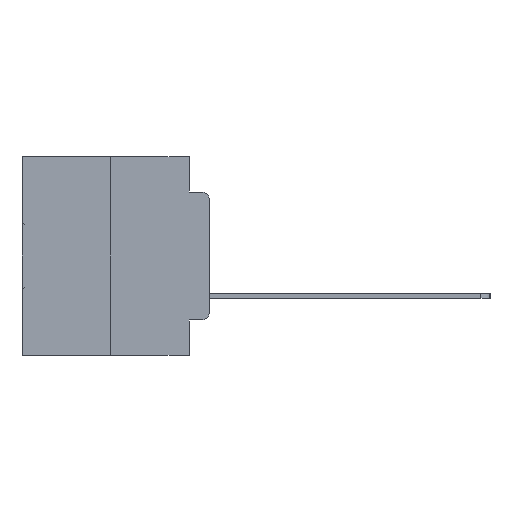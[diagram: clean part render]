
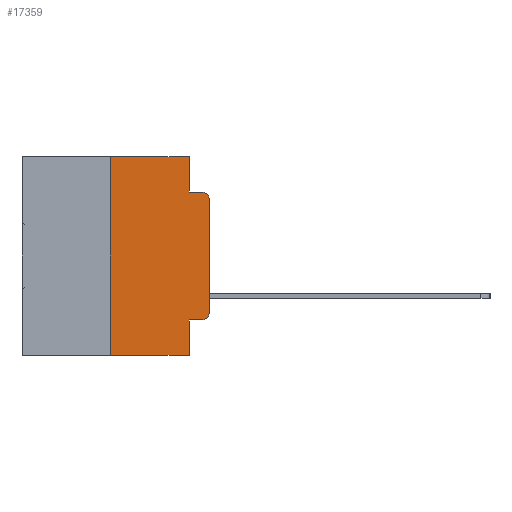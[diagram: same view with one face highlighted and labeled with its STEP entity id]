
A CAD part, left-side view. The second image highlights one B-rep face of the part: STEP entity #17359.
In plain terms, the highlighted planar face has unit normal (-1, 0, 0).
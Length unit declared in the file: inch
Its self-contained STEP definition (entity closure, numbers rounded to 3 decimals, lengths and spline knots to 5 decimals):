
#674 = EDGE_CURVE ( 'NONE', #1802, #11929, #8612, .T. ) ;
#1368 = CARTESIAN_POINT ( 'NONE',  ( 0., 0.473, 0. ) ) ;
#1500 = CARTESIAN_POINT ( 'NONE',  ( 0., 0.25, 0. ) ) ;
#1729 = CARTESIAN_POINT ( 'NONE',  ( 0., 0.02, -0.1085 ) ) ;
#1802 = VERTEX_POINT ( 'NONE', #5630 ) ;
#1898 = VERTEX_POINT ( 'NONE', #11949 ) ;
#2174 = VERTEX_POINT ( 'NONE', #17420 ) ;
#2184 = ORIENTED_EDGE ( 'NONE', *, *, #27439, .F. ) ;
#2606 = VECTOR ( 'NONE', #14664, 39.37008 ) ;
#2814 = CARTESIAN_POINT ( 'NONE',  ( 0., 0.051, 0. ) ) ;
#2825 = ORIENTED_EDGE ( 'NONE', *, *, #14005, .F. ) ;
#3076 = CARTESIAN_POINT ( 'NONE',  ( 0., 0.051, -0.0885 ) ) ;
#3479 = VERTEX_POINT ( 'NONE', #28810 ) ;
#3806 = DIRECTION ( 'NONE',  ( 0., 0., -1. ) ) ;
#3943 = CIRCLE ( 'NONE', #24293, 0.02 ) ;
#4190 = DIRECTION ( 'NONE',  ( 0., 0., -1. ) ) ;
#4586 = EDGE_LOOP ( 'NONE', ( #26610, #17280, #2184, #21077, #2825, #12825, #13904, #21691, #17058, #21719 ) ) ;
#5586 = EDGE_CURVE ( 'NONE', #2174, #3479, #14502, .T. ) ;
#5630 = CARTESIAN_POINT ( 'NONE',  ( 0., 0.051, 0. ) ) ;
#6477 = LINE ( 'NONE', #20617, #30353 ) ;
#6943 = CARTESIAN_POINT ( 'NONE',  ( 0., 0.051, -0.0885 ) ) ;
#7301 = LINE ( 'NONE', #1500, #25558 ) ;
#7636 = DIRECTION ( 'NONE',  ( -1., 0., 0. ) ) ;
#8612 = LINE ( 'NONE', #2814, #20515 ) ;
#8879 = DIRECTION ( 'NONE',  ( 0., 0., 1. ) ) ;
#9117 = LINE ( 'NONE', #26446, #2606 ) ;
#9449 = CARTESIAN_POINT ( 'NONE',  ( 0., 0.051, 0. ) ) ;
#9705 = DIRECTION ( 'NONE',  ( 0., 0., 1. ) ) ;
#9965 = CARTESIAN_POINT ( 'NONE',  ( 0., 0.051, -0.5 ) ) ;
#10121 = EDGE_CURVE ( 'NONE', #19025, #30671, #3943, .T. ) ;
#10671 = VERTEX_POINT ( 'NONE', #9965 ) ;
#11039 = PLANE ( 'NONE',  #29681 ) ;
#11929 = VERTEX_POINT ( 'NONE', #3076 ) ;
#11949 = CARTESIAN_POINT ( 'NONE',  ( 0., 0.25, 0. ) ) ;
#11959 = DIRECTION ( 'NONE',  ( 0., 0., -1. ) ) ;
#12344 = EDGE_CURVE ( 'NONE', #26546, #10671, #24048, .T. ) ;
#12825 = ORIENTED_EDGE ( 'NONE', *, *, #25640, .F. ) ;
#13904 = ORIENTED_EDGE ( 'NONE', *, *, #20750, .T. ) ;
#14005 = EDGE_CURVE ( 'NONE', #1898, #1802, #9117, .T. ) ;
#14502 = CIRCLE ( 'NONE', #23609, 0.02 ) ;
#14618 = CARTESIAN_POINT ( 'NONE',  ( 0., 0.051, -0.4115 ) ) ;
#14664 = DIRECTION ( 'NONE',  ( 0., -1., 0. ) ) ;
#16967 = CARTESIAN_POINT ( 'NONE',  ( 0., 0.051, -0.4115 ) ) ;
#17058 = ORIENTED_EDGE ( 'NONE', *, *, #23199, .T. ) ;
#17280 = ORIENTED_EDGE ( 'NONE', *, *, #5586, .T. ) ;
#17353 = VECTOR ( 'NONE', #9705, 39.37008 ) ;
#17359 = ADVANCED_FACE ( 'NONE', ( #29106 ), #11039, .F. ) ;
#17420 = CARTESIAN_POINT ( 'NONE',  ( 0., 0., -0.1085 ) ) ;
#18228 = DIRECTION ( 'NONE',  ( 1., 0., 0. ) ) ;
#18255 = DIRECTION ( 'NONE',  ( 0., -1., 0. ) ) ;
#18411 = VECTOR ( 'NONE', #28417, 39.37008 ) ;
#18585 = DIRECTION ( 'NONE',  ( -1., 0., 0. ) ) ;
#19025 = VERTEX_POINT ( 'NONE', #27787 ) ;
#19155 = LINE ( 'NONE', #6943, #18411 ) ;
#19171 = CARTESIAN_POINT ( 'NONE',  ( 0., 0., 0. ) ) ;
#20515 = VECTOR ( 'NONE', #30918, 39.37008 ) ;
#20617 = CARTESIAN_POINT ( 'NONE',  ( 0., 0.473, -0.5 ) ) ;
#20750 = EDGE_CURVE ( 'NONE', #27465, #10671, #6477, .T. ) ;
#20982 = EDGE_CURVE ( 'NONE', #30671, #2174, #23634, .T. ) ;
#21077 = ORIENTED_EDGE ( 'NONE', *, *, #674, .F. ) ;
#21439 = CARTESIAN_POINT ( 'NONE',  ( 0., 0.25, -0.5 ) ) ;
#21691 = ORIENTED_EDGE ( 'NONE', *, *, #12344, .F. ) ;
#21719 = ORIENTED_EDGE ( 'NONE', *, *, #10121, .T. ) ;
#21899 = CARTESIAN_POINT ( 'NONE',  ( 0., 0.02, -0.3915 ) ) ;
#22350 = VECTOR ( 'NONE', #28808, 39.37008 ) ;
#23092 = LINE ( 'NONE', #14618, #22350 ) ;
#23199 = EDGE_CURVE ( 'NONE', #26546, #19025, #23092, .T. ) ;
#23609 = AXIS2_PLACEMENT_3D ( 'NONE', #1729, #18585, #4190 ) ;
#23634 = LINE ( 'NONE', #19171, #17353 ) ;
#24048 = LINE ( 'NONE', #9449, #29645 ) ;
#24280 = DIRECTION ( 'NONE',  ( 0., 0., -1. ) ) ;
#24293 = AXIS2_PLACEMENT_3D ( 'NONE', #21899, #7636, #24280 ) ;
#25558 = VECTOR ( 'NONE', #8879, 39.37008 ) ;
#25640 = EDGE_CURVE ( 'NONE', #27465, #1898, #7301, .T. ) ;
#26418 = CARTESIAN_POINT ( 'NONE',  ( 0., 0., -0.3915 ) ) ;
#26446 = CARTESIAN_POINT ( 'NONE',  ( 0., 0.473, 0. ) ) ;
#26546 = VERTEX_POINT ( 'NONE', #16967 ) ;
#26610 = ORIENTED_EDGE ( 'NONE', *, *, #20982, .T. ) ;
#27439 = EDGE_CURVE ( 'NONE', #11929, #3479, #19155, .T. ) ;
#27465 = VERTEX_POINT ( 'NONE', #21439 ) ;
#27787 = CARTESIAN_POINT ( 'NONE',  ( 0., 0.02, -0.4115 ) ) ;
#28417 = DIRECTION ( 'NONE',  ( 0., -1., 0. ) ) ;
#28808 = DIRECTION ( 'NONE',  ( 0., -1., 0. ) ) ;
#28810 = CARTESIAN_POINT ( 'NONE',  ( 0., 0.02, -0.0885 ) ) ;
#29106 = FACE_OUTER_BOUND ( 'NONE', #4586, .T. ) ;
#29645 = VECTOR ( 'NONE', #11959, 39.37008 ) ;
#29681 = AXIS2_PLACEMENT_3D ( 'NONE', #1368, #18228, #3806 ) ;
#30353 = VECTOR ( 'NONE', #18255, 39.37008 ) ;
#30671 = VERTEX_POINT ( 'NONE', #26418 ) ;
#30918 = DIRECTION ( 'NONE',  ( 0., 0., -1. ) ) ;
